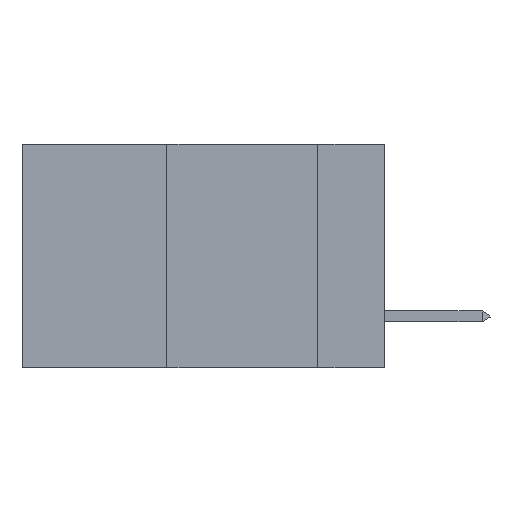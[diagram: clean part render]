
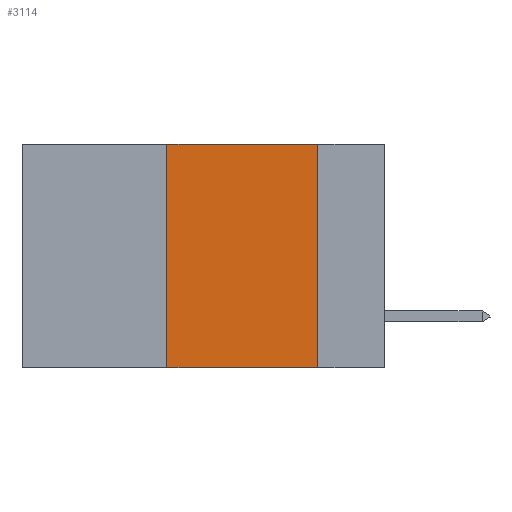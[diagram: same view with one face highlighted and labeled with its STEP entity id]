
A CAD part, left-side view. The second image highlights one B-rep face of the part: STEP entity #3114.
In plain terms, the highlighted planar face has unit normal (-1, 0, 0).
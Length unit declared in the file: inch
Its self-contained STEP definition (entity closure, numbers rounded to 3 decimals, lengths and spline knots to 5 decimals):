
#190 = CARTESIAN_POINT ( 'NONE',  ( 0., 0.6, 0. ) ) ;
#714 = LINE ( 'NONE', #9854, #10744 ) ;
#765 = DIRECTION ( 'NONE',  ( 0., 0., 1. ) ) ;
#1263 = DIRECTION ( 'NONE',  ( 0., -1., 0. ) ) ;
#1408 = EDGE_CURVE ( 'NONE', #11949, #8568, #7376, .T. ) ;
#1729 = EDGE_CURVE ( 'NONE', #11949, #3198, #6829, .T. ) ;
#3114 = ADVANCED_FACE ( 'NONE', ( #12821 ), #7761, .F. ) ;
#3198 = VERTEX_POINT ( 'NONE', #6861 ) ;
#4131 = CARTESIAN_POINT ( 'NONE',  ( 0., 0.36, 0. ) ) ;
#4317 = ORIENTED_EDGE ( 'NONE', *, *, #1408, .T. ) ;
#4719 = EDGE_LOOP ( 'NONE', ( #12813, #8471, #5389, #4317 ) ) ;
#4792 = EDGE_CURVE ( 'NONE', #8323, #8568, #714, .T. ) ;
#5389 = ORIENTED_EDGE ( 'NONE', *, *, #1729, .F. ) ;
#6390 = CARTESIAN_POINT ( 'NONE',  ( 0., 0.6, 0. ) ) ;
#6413 = CARTESIAN_POINT ( 'NONE',  ( 0., 0.11, -0.37 ) ) ;
#6549 = DIRECTION ( 'NONE',  ( 0., 0., -1. ) ) ;
#6641 = VECTOR ( 'NONE', #1263, 39.37008 ) ;
#6829 = LINE ( 'NONE', #4131, #9913 ) ;
#6861 = CARTESIAN_POINT ( 'NONE',  ( 0., 0.36, 0. ) ) ;
#7376 = LINE ( 'NONE', #12956, #6641 ) ;
#7559 = DIRECTION ( 'NONE',  ( 1., 0., 0. ) ) ;
#7761 = PLANE ( 'NONE',  #12334 ) ;
#7836 = EDGE_CURVE ( 'NONE', #3198, #8323, #12537, .T. ) ;
#8323 = VERTEX_POINT ( 'NONE', #12958 ) ;
#8332 = DIRECTION ( 'NONE',  ( 0., -1., 0. ) ) ;
#8471 = ORIENTED_EDGE ( 'NONE', *, *, #7836, .F. ) ;
#8568 = VERTEX_POINT ( 'NONE', #6413 ) ;
#9854 = CARTESIAN_POINT ( 'NONE',  ( 0., 0.11, 0. ) ) ;
#9895 = DIRECTION ( 'NONE',  ( 0., 0., -1. ) ) ;
#9913 = VECTOR ( 'NONE', #765, 39.37008 ) ;
#10744 = VECTOR ( 'NONE', #6549, 39.37008 ) ;
#11949 = VERTEX_POINT ( 'NONE', #13496 ) ;
#12334 = AXIS2_PLACEMENT_3D ( 'NONE', #6390, #7559, #9895 ) ;
#12537 = LINE ( 'NONE', #190, #14155 ) ;
#12813 = ORIENTED_EDGE ( 'NONE', *, *, #4792, .F. ) ;
#12821 = FACE_OUTER_BOUND ( 'NONE', #4719, .T. ) ;
#12956 = CARTESIAN_POINT ( 'NONE',  ( 0., 0.6, -0.37 ) ) ;
#12958 = CARTESIAN_POINT ( 'NONE',  ( 0., 0.11, 0. ) ) ;
#13496 = CARTESIAN_POINT ( 'NONE',  ( 0., 0.36, -0.37 ) ) ;
#14155 = VECTOR ( 'NONE', #8332, 39.37008 ) ;
